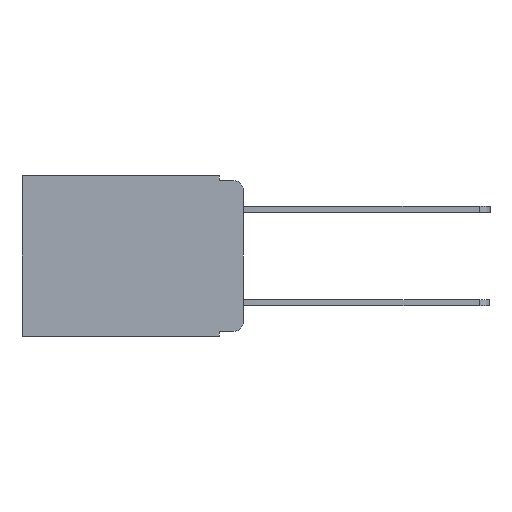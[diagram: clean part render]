
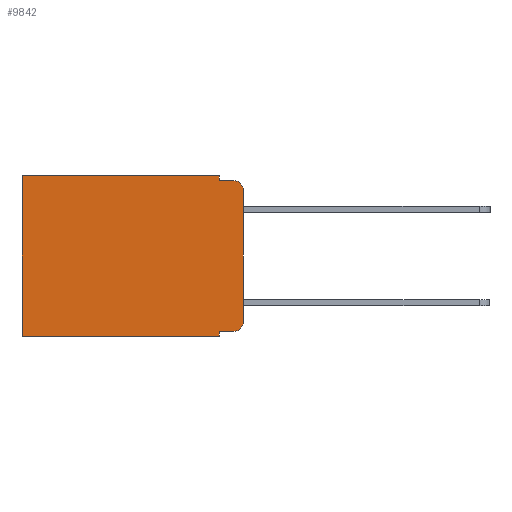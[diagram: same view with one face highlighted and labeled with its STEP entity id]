
A CAD part, left-side view. The second image highlights one B-rep face of the part: STEP entity #9842.
In plain terms, the highlighted planar face has unit normal (-1, 0, 0).
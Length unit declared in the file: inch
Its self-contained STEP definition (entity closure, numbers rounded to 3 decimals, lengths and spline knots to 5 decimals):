
#439 = LINE ( 'NONE', #8777, #8268 ) ;
#472 = LINE ( 'NONE', #6770, #11352 ) ;
#478 = EDGE_CURVE ( 'NONE', #5772, #11648, #8447, .T. ) ;
#702 = ORIENTED_EDGE ( 'NONE', *, *, #5357, .T. ) ;
#732 = AXIS2_PLACEMENT_3D ( 'NONE', #1881, #8621, #2932 ) ;
#1014 = VERTEX_POINT ( 'NONE', #10850 ) ;
#1224 = CARTESIAN_POINT ( 'NONE',  ( 0.298, 0.02, -0.333 ) ) ;
#1345 = VERTEX_POINT ( 'NONE', #8802 ) ;
#1698 = LINE ( 'NONE', #1911, #4148 ) ;
#1815 = CARTESIAN_POINT ( 'NONE',  ( 0.298, 0.02, -0.01 ) ) ;
#1867 = CARTESIAN_POINT ( 'NONE',  ( 0.298, 0.051, 0. ) ) ;
#1881 = CARTESIAN_POINT ( 'NONE',  ( 0.298, 0.02, -0.03 ) ) ;
#1911 = CARTESIAN_POINT ( 'NONE',  ( 0.298, 0.051, 0. ) ) ;
#1957 = DIRECTION ( 'NONE',  ( 0., -1., 0. ) ) ;
#2426 = EDGE_LOOP ( 'NONE', ( #3965, #2825, #5617, #8480, #5903, #3335, #5164, #9428, #702, #11017 ) ) ;
#2624 = VERTEX_POINT ( 'NONE', #1224 ) ;
#2825 = ORIENTED_EDGE ( 'NONE', *, *, #8792, .T. ) ;
#2873 = CARTESIAN_POINT ( 'NONE',  ( 0.298, 0.051, -0.333 ) ) ;
#2872 = PLANE ( 'NONE',  #6772 ) ;
#2888 = VERTEX_POINT ( 'NONE', #1815 ) ;
#2932 = DIRECTION ( 'NONE',  ( 0., 0., -1. ) ) ;
#3174 = VERTEX_POINT ( 'NONE', #6550 ) ;
#3335 = ORIENTED_EDGE ( 'NONE', *, *, #5373, .T. ) ;
#3444 = VECTOR ( 'NONE', #3500, 39.37008 ) ;
#3500 = DIRECTION ( 'NONE',  ( 0., 1., 0. ) ) ;
#3631 = CARTESIAN_POINT ( 'NONE',  ( 0.298, 0.473, 0. ) ) ;
#3932 = DIRECTION ( 'NONE',  ( 1., 0., 0. ) ) ;
#3965 = ORIENTED_EDGE ( 'NONE', *, *, #8652, .F. ) ;
#3981 = DIRECTION ( 'NONE',  ( -1., 0., 0. ) ) ;
#4148 = VECTOR ( 'NONE', #9495, 39.37008 ) ;
#4276 = CARTESIAN_POINT ( 'NONE',  ( 0.298, 0., -0.343 ) ) ;
#4476 = VECTOR ( 'NONE', #11947, 39.37008 ) ;
#4791 = VERTEX_POINT ( 'NONE', #8282 ) ;
#5164 = ORIENTED_EDGE ( 'NONE', *, *, #478, .F. ) ;
#5165 = LINE ( 'NONE', #2873, #7556 ) ;
#5357 = EDGE_CURVE ( 'NONE', #4791, #2624, #5165, .T. ) ;
#5370 = EDGE_CURVE ( 'NONE', #2624, #3174, #7291, .T. ) ;
#5371 = EDGE_CURVE ( 'NONE', #4791, #5772, #11526, .T. ) ;
#5373 = EDGE_CURVE ( 'NONE', #7955, #11648, #9557, .T. ) ;
#5388 = EDGE_CURVE ( 'NONE', #5830, #1014, #1698, .T. ) ;
#5617 = ORIENTED_EDGE ( 'NONE', *, *, #9912, .F. ) ;
#5772 = VERTEX_POINT ( 'NONE', #11545 ) ;
#5830 = VERTEX_POINT ( 'NONE', #10788 ) ;
#5903 = ORIENTED_EDGE ( 'NONE', *, *, #10997, .T. ) ;
#6550 = CARTESIAN_POINT ( 'NONE',  ( 0.298, 0., -0.313 ) ) ;
#6770 = CARTESIAN_POINT ( 'NONE',  ( 0.298, 0., 0. ) ) ;
#6772 = AXIS2_PLACEMENT_3D ( 'NONE', #11089, #3932, #10263 ) ;
#6799 = CARTESIAN_POINT ( 'NONE',  ( 0.298, 0.473, -0.343 ) ) ;
#6868 = DIRECTION ( 'NONE',  ( 0., 0., -1. ) ) ;
#7043 = DIRECTION ( 'NONE',  ( 0., 1., 0. ) ) ;
#7291 = CIRCLE ( 'NONE', #7683, 0.02 ) ;
#7556 = VECTOR ( 'NONE', #10264, 39.37008 ) ;
#7612 = VECTOR ( 'NONE', #1957, 39.37008 ) ;
#7683 = AXIS2_PLACEMENT_3D ( 'NONE', #9465, #3981, #10300 ) ;
#7955 = VERTEX_POINT ( 'NONE', #3631 ) ;
#8138 = FACE_OUTER_BOUND ( 'NONE', #2426, .T. ) ;
#8268 = VECTOR ( 'NONE', #7043, 39.37008 ) ;
#8282 = CARTESIAN_POINT ( 'NONE',  ( 0.298, 0.051, -0.333 ) ) ;
#8447 = LINE ( 'NONE', #4276, #3444 ) ;
#8480 = ORIENTED_EDGE ( 'NONE', *, *, #5388, .F. ) ;
#8499 = DIRECTION ( 'NONE',  ( 0., 0., -1. ) ) ;
#8621 = DIRECTION ( 'NONE',  ( -1., 0., 0. ) ) ;
#8652 = EDGE_CURVE ( 'NONE', #1345, #3174, #472, .T. ) ;
#8685 = CARTESIAN_POINT ( 'NONE',  ( 0.298, 0.051, -0.01 ) ) ;
#8777 = CARTESIAN_POINT ( 'NONE',  ( 0.298, 0., 0. ) ) ;
#8792 = EDGE_CURVE ( 'NONE', #1345, #2888, #10031, .T. ) ;
#8802 = CARTESIAN_POINT ( 'NONE',  ( 0.298, 0., -0.03 ) ) ;
#9299 = VECTOR ( 'NONE', #6868, 39.37008 ) ;
#9428 = ORIENTED_EDGE ( 'NONE', *, *, #5371, .F. ) ;
#9465 = CARTESIAN_POINT ( 'NONE',  ( 0.298, 0.02, -0.313 ) ) ;
#9495 = DIRECTION ( 'NONE',  ( 0., 0., -1. ) ) ;
#9557 = LINE ( 'NONE', #11170, #4476 ) ;
#9842 = ADVANCED_FACE ( 'NONE', ( #8138 ), #2872, .F. ) ;
#9912 = EDGE_CURVE ( 'NONE', #1014, #2888, #11814, .T. ) ;
#10031 = CIRCLE ( 'NONE', #732, 0.02 ) ;
#10264 = DIRECTION ( 'NONE',  ( 0., -1., 0. ) ) ;
#10263 = DIRECTION ( 'NONE',  ( 0., 0., -1. ) ) ;
#10300 = DIRECTION ( 'NONE',  ( 0., 0., -1. ) ) ;
#10788 = CARTESIAN_POINT ( 'NONE',  ( 0.298, 0.051, 0. ) ) ;
#10850 = CARTESIAN_POINT ( 'NONE',  ( 0.298, 0.051, -0.01 ) ) ;
#10997 = EDGE_CURVE ( 'NONE', #5830, #7955, #439, .T. ) ;
#11017 = ORIENTED_EDGE ( 'NONE', *, *, #5370, .T. ) ;
#11089 = CARTESIAN_POINT ( 'NONE',  ( 0.298, 0., 0. ) ) ;
#11170 = CARTESIAN_POINT ( 'NONE',  ( 0.298, 0.473, 0. ) ) ;
#11352 = VECTOR ( 'NONE', #8499, 39.37008 ) ;
#11526 = LINE ( 'NONE', #1867, #9299 ) ;
#11545 = CARTESIAN_POINT ( 'NONE',  ( 0.298, 0.051, -0.343 ) ) ;
#11648 = VERTEX_POINT ( 'NONE', #6799 ) ;
#11814 = LINE ( 'NONE', #8685, #7612 ) ;
#11947 = DIRECTION ( 'NONE',  ( 0., 0., -1. ) ) ;
